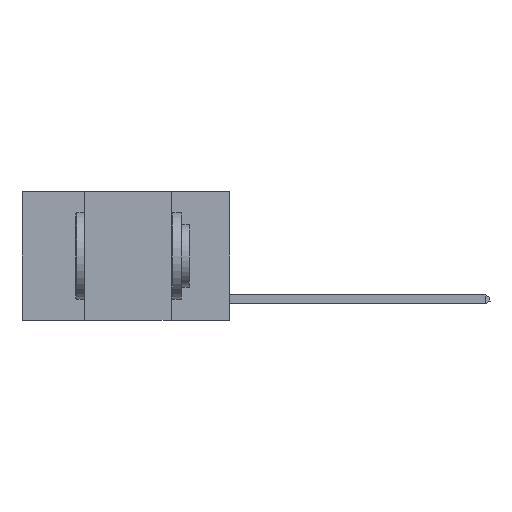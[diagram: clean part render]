
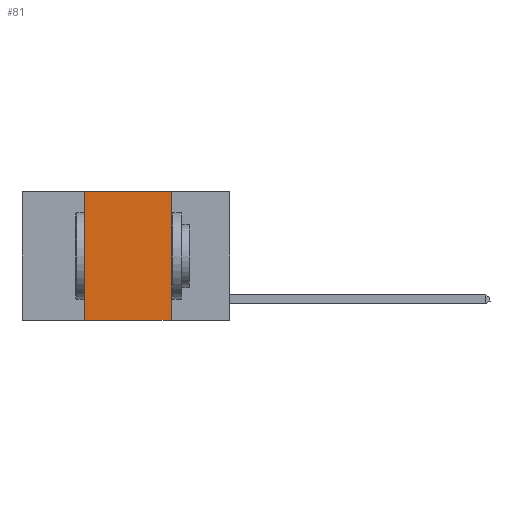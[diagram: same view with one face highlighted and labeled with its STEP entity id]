
A CAD part, left-side view. The second image highlights one B-rep face of the part: STEP entity #81.
In plain terms, the highlighted planar face has unit normal (-1, 0, 0).
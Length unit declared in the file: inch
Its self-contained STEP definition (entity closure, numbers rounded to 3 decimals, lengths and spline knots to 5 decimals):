
#28 = VERTEX_POINT ( 'NONE', #7546 ) ;
#81 = ADVANCED_FACE ( 'NONE', ( #19233 ), #17009, .F. ) ;
#1216 = CARTESIAN_POINT ( 'NONE',  ( 0., 0.42, 0. ) ) ;
#2475 = EDGE_CURVE ( 'NONE', #11388, #18901, #7707, .T. ) ;
#2675 = EDGE_CURVE ( 'NONE', #18901, #4533, #21723, .T. ) ;
#4533 = VERTEX_POINT ( 'NONE', #12875 ) ;
#4868 = LINE ( 'NONE', #19025, #18181 ) ;
#7189 = ORIENTED_EDGE ( 'NONE', *, *, #2475, .F. ) ;
#7546 = CARTESIAN_POINT ( 'NONE',  ( 0., 0.17, -0.37 ) ) ;
#7707 = LINE ( 'NONE', #18017, #20917 ) ;
#8371 = LINE ( 'NONE', #9580, #16521 ) ;
#8615 = DIRECTION ( 'NONE',  ( 1., 0., 0. ) ) ;
#9397 = ORIENTED_EDGE ( 'NONE', *, *, #2675, .F. ) ;
#9580 = CARTESIAN_POINT ( 'NONE',  ( 0., 0.6, -0.37 ) ) ;
#10507 = CARTESIAN_POINT ( 'NONE',  ( 0., 0.6, 0. ) ) ;
#11388 = VERTEX_POINT ( 'NONE', #18846 ) ;
#11598 = DIRECTION ( 'NONE',  ( 0., -1., 0. ) ) ;
#12307 = EDGE_CURVE ( 'NONE', #11388, #28, #8371, .T. ) ;
#12507 = ORIENTED_EDGE ( 'NONE', *, *, #21072, .F. ) ;
#12875 = CARTESIAN_POINT ( 'NONE',  ( 0., 0.17, 0. ) ) ;
#13009 = DIRECTION ( 'NONE',  ( 0., -1., 0. ) ) ;
#13881 = DIRECTION ( 'NONE',  ( 0., 0., -1. ) ) ;
#14612 = ORIENTED_EDGE ( 'NONE', *, *, #12307, .T. ) ;
#15121 = CARTESIAN_POINT ( 'NONE',  ( 0., 0.6, 0. ) ) ;
#16427 = AXIS2_PLACEMENT_3D ( 'NONE', #10507, #8615, #13881 ) ;
#16521 = VECTOR ( 'NONE', #13009, 39.37008 ) ;
#17009 = PLANE ( 'NONE',  #16427 ) ;
#17139 = EDGE_LOOP ( 'NONE', ( #12507, #9397, #7189, #14612 ) ) ;
#17167 = VECTOR ( 'NONE', #11598, 39.37008 ) ;
#18017 = CARTESIAN_POINT ( 'NONE',  ( 0., 0.42, 0. ) ) ;
#18181 = VECTOR ( 'NONE', #20716, 39.37008 ) ;
#18846 = CARTESIAN_POINT ( 'NONE',  ( 0., 0.42, -0.37 ) ) ;
#18901 = VERTEX_POINT ( 'NONE', #1216 ) ;
#19025 = CARTESIAN_POINT ( 'NONE',  ( 0., 0.17, 0. ) ) ;
#19233 = FACE_OUTER_BOUND ( 'NONE', #17139, .T. ) ;
#19729 = DIRECTION ( 'NONE',  ( 0., 0., 1. ) ) ;
#20716 = DIRECTION ( 'NONE',  ( 0., 0., -1. ) ) ;
#20917 = VECTOR ( 'NONE', #19729, 39.37008 ) ;
#21072 = EDGE_CURVE ( 'NONE', #4533, #28, #4868, .T. ) ;
#21723 = LINE ( 'NONE', #15121, #17167 ) ;
